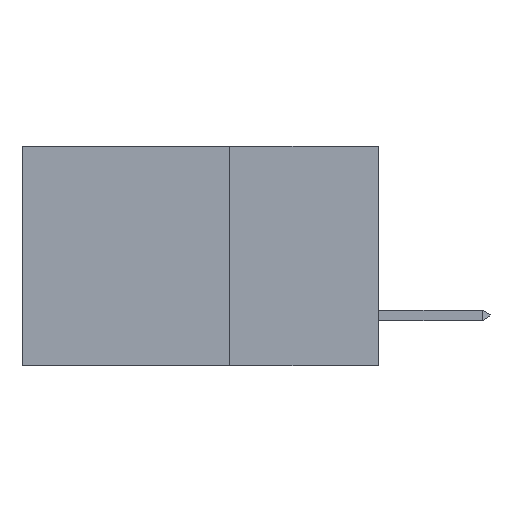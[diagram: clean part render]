
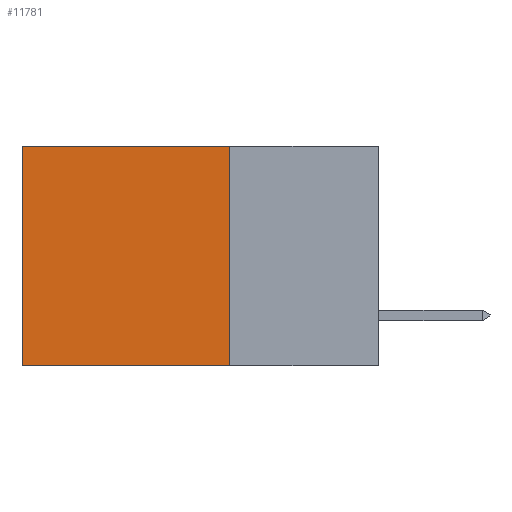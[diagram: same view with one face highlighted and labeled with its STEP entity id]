
A CAD part, left-side view. The second image highlights one B-rep face of the part: STEP entity #11781.
In plain terms, the highlighted planar face has unit normal (-1, 0, 0).
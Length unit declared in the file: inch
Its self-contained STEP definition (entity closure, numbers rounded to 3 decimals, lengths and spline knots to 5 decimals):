
#48 = VERTEX_POINT ( 'NONE', #7892 ) ;
#727 = DIRECTION ( 'NONE',  ( 0., 0., -1. ) ) ;
#857 = DIRECTION ( 'NONE',  ( 0., 1., 0. ) ) ;
#1254 = ORIENTED_EDGE ( 'NONE', *, *, #6586, .F. ) ;
#1455 = EDGE_LOOP ( 'NONE', ( #4798, #3059, #1254, #2826 ) ) ;
#1752 = LINE ( 'NONE', #9028, #11142 ) ;
#1949 = VECTOR ( 'NONE', #6459, 39.37008 ) ;
#2029 = VECTOR ( 'NONE', #857, 39.37008 ) ;
#2249 = CARTESIAN_POINT ( 'NONE',  ( 0.2615, 0.6, 0. ) ) ;
#2336 = CARTESIAN_POINT ( 'NONE',  ( 0.2615, 0.25, -0.37 ) ) ;
#2826 = ORIENTED_EDGE ( 'NONE', *, *, #4331, .T. ) ;
#2967 = EDGE_CURVE ( 'NONE', #5236, #48, #4421, .T. ) ;
#3059 = ORIENTED_EDGE ( 'NONE', *, *, #6348, .F. ) ;
#3583 = VECTOR ( 'NONE', #727, 39.37008 ) ;
#3862 = CARTESIAN_POINT ( 'NONE',  ( 0.2615, 0.25, -0.37 ) ) ;
#4331 = EDGE_CURVE ( 'NONE', #10266, #5236, #12338, .T. ) ;
#4421 = LINE ( 'NONE', #5448, #1949 ) ;
#4798 = ORIENTED_EDGE ( 'NONE', *, *, #2967, .T. ) ;
#4902 = CARTESIAN_POINT ( 'NONE',  ( 0.2615, 0.25, 0. ) ) ;
#4909 = FACE_OUTER_BOUND ( 'NONE', #1455, .T. ) ;
#5236 = VERTEX_POINT ( 'NONE', #2249 ) ;
#5448 = CARTESIAN_POINT ( 'NONE',  ( 0.2615, 0.6, -0.37 ) ) ;
#5591 = AXIS2_PLACEMENT_3D ( 'NONE', #9131, #11095, #5928 ) ;
#5928 = DIRECTION ( 'NONE',  ( 0., 0., -1. ) ) ;
#6348 = EDGE_CURVE ( 'NONE', #12218, #48, #1752, .T. ) ;
#6459 = DIRECTION ( 'NONE',  ( 0., 0., -1. ) ) ;
#6586 = EDGE_CURVE ( 'NONE', #10266, #12218, #12140, .T. ) ;
#7892 = CARTESIAN_POINT ( 'NONE',  ( 0.2615, 0.6, -0.37 ) ) ;
#9028 = CARTESIAN_POINT ( 'NONE',  ( 0.2615, 0.25, -0.37 ) ) ;
#9131 = CARTESIAN_POINT ( 'NONE',  ( 0.2615, 0.25, -0.37 ) ) ;
#10266 = VERTEX_POINT ( 'NONE', #11447 ) ;
#11095 = DIRECTION ( 'NONE',  ( 1., 0., 0. ) ) ;
#11142 = VECTOR ( 'NONE', #11193, 39.37008 ) ;
#11193 = DIRECTION ( 'NONE',  ( 0., 1., 0. ) ) ;
#11447 = CARTESIAN_POINT ( 'NONE',  ( 0.2615, 0.25, 0. ) ) ;
#11781 = ADVANCED_FACE ( 'NONE', ( #4909 ), #13086, .F. ) ;
#12140 = LINE ( 'NONE', #2336, #3583 ) ;
#12218 = VERTEX_POINT ( 'NONE', #3862 ) ;
#12338 = LINE ( 'NONE', #4902, #2029 ) ;
#13086 = PLANE ( 'NONE',  #5591 ) ;
